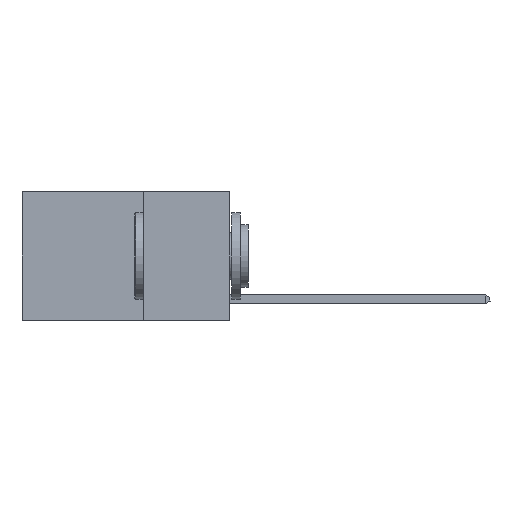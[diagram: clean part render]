
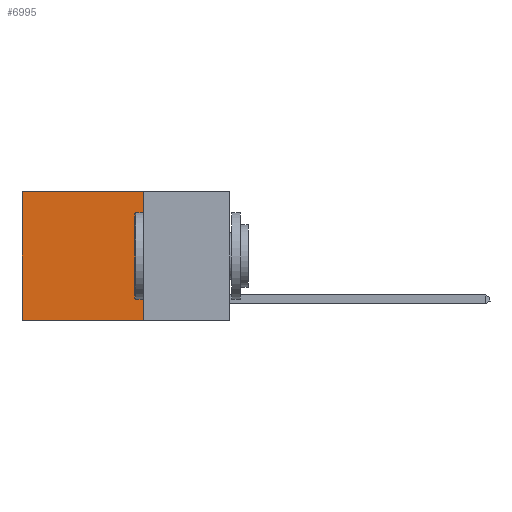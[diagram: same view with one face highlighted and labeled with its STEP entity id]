
A CAD part, left-side view. The second image highlights one B-rep face of the part: STEP entity #6995.
In plain terms, the highlighted planar face has unit normal (-1, 0, 0).
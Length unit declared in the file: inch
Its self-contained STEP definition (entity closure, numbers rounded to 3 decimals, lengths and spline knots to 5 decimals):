
#214 = LINE ( 'NONE', #14774, #4724 ) ;
#1397 = DIRECTION ( 'NONE',  ( 1., 0., 0. ) ) ;
#2254 = VECTOR ( 'NONE', #20151, 39.37008 ) ;
#2424 = CARTESIAN_POINT ( 'NONE',  ( 0.2625, 0.25, 0. ) ) ;
#2425 = LINE ( 'NONE', #2424, #17631 ) ;
#2667 = ORIENTED_EDGE ( 'NONE', *, *, #15790, .T. ) ;
#4724 = VECTOR ( 'NONE', #16681, 39.37008 ) ;
#4892 = DIRECTION ( 'NONE',  ( 0., 1., 0. ) ) ;
#6873 = AXIS2_PLACEMENT_3D ( 'NONE', #18518, #1397, #14772 ) ;
#6995 = ADVANCED_FACE ( 'NONE', ( #16752 ), #22388, .F. ) ;
#7207 = EDGE_CURVE ( 'NONE', #15360, #15572, #2425, .T. ) ;
#7224 = ORIENTED_EDGE ( 'NONE', *, *, #12981, .T. ) ;
#7297 = LINE ( 'NONE', #16209, #2254 ) ;
#8323 = CARTESIAN_POINT ( 'NONE',  ( 0.2625, 0.6, -0.37 ) ) ;
#8656 = LINE ( 'NONE', #18231, #19413 ) ;
#11845 = CARTESIAN_POINT ( 'NONE',  ( 0.2625, 0.25, -0.37 ) ) ;
#12981 = EDGE_CURVE ( 'NONE', #15360, #18737, #8656, .T. ) ;
#13840 = DIRECTION ( 'NONE',  ( 0., 0., -1. ) ) ;
#14291 = ORIENTED_EDGE ( 'NONE', *, *, #19330, .F. ) ;
#14772 = DIRECTION ( 'NONE',  ( 0., 0., -1. ) ) ;
#14774 = CARTESIAN_POINT ( 'NONE',  ( 0.2625, 0.25, -0.37 ) ) ;
#15360 = VERTEX_POINT ( 'NONE', #18891 ) ;
#15572 = VERTEX_POINT ( 'NONE', #11845 ) ;
#15790 = EDGE_CURVE ( 'NONE', #18737, #21995, #7297, .T. ) ;
#15888 = ORIENTED_EDGE ( 'NONE', *, *, #7207, .F. ) ;
#16209 = CARTESIAN_POINT ( 'NONE',  ( 0.2625, 0.6, 0. ) ) ;
#16681 = DIRECTION ( 'NONE',  ( 0., 1., 0. ) ) ;
#16752 = FACE_OUTER_BOUND ( 'NONE', #20535, .T. ) ;
#17631 = VECTOR ( 'NONE', #13840, 39.37008 ) ;
#18231 = CARTESIAN_POINT ( 'NONE',  ( 0.2625, 0.25, 0. ) ) ;
#18518 = CARTESIAN_POINT ( 'NONE',  ( 0.2625, 0.25, 0. ) ) ;
#18737 = VERTEX_POINT ( 'NONE', #22412 ) ;
#18891 = CARTESIAN_POINT ( 'NONE',  ( 0.2625, 0.25, 0. ) ) ;
#19330 = EDGE_CURVE ( 'NONE', #15572, #21995, #214, .T. ) ;
#19413 = VECTOR ( 'NONE', #4892, 39.37008 ) ;
#20151 = DIRECTION ( 'NONE',  ( 0., 0., -1. ) ) ;
#20535 = EDGE_LOOP ( 'NONE', ( #2667, #14291, #15888, #7224 ) ) ;
#21995 = VERTEX_POINT ( 'NONE', #8323 ) ;
#22388 = PLANE ( 'NONE',  #6873 ) ;
#22412 = CARTESIAN_POINT ( 'NONE',  ( 0.2625, 0.6, 0. ) ) ;
